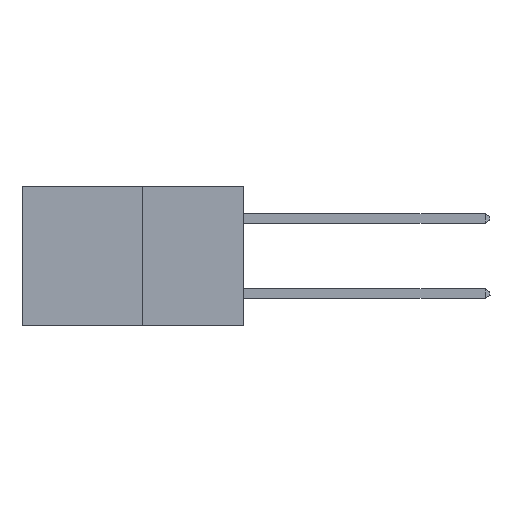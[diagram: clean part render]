
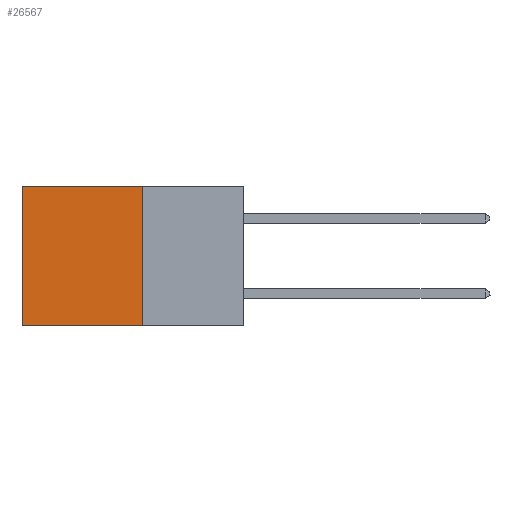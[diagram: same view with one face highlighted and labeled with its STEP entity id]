
A CAD part, left-side view. The second image highlights one B-rep face of the part: STEP entity #26567.
In plain terms, the highlighted planar face has unit normal (-1, 0, 0).
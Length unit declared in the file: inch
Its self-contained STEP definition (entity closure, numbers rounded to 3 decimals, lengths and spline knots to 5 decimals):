
#114 = FACE_OUTER_BOUND ( 'NONE', #4023, .T. ) ;
#554 = EDGE_CURVE ( 'NONE', #22912, #1850, #18819, .T. ) ;
#1509 = CARTESIAN_POINT ( 'NONE',  ( 0.277, 0.59, -0.37 ) ) ;
#1777 = CARTESIAN_POINT ( 'NONE',  ( 0.277, 0.27, -0.37 ) ) ;
#1818 = VERTEX_POINT ( 'NONE', #24391 ) ;
#1850 = VERTEX_POINT ( 'NONE', #26605 ) ;
#2581 = ORIENTED_EDGE ( 'NONE', *, *, #26388, .T. ) ;
#4023 = EDGE_LOOP ( 'NONE', ( #2581, #30947, #9763, #32124 ) ) ;
#4091 = VERTEX_POINT ( 'NONE', #1777 ) ;
#4722 = DIRECTION ( 'NONE',  ( 1., 0., 0. ) ) ;
#4910 = VECTOR ( 'NONE', #6625, 39.37008 ) ;
#5679 = CARTESIAN_POINT ( 'NONE',  ( 0.277, 0.27, 0. ) ) ;
#6625 = DIRECTION ( 'NONE',  ( 0., 0., -1. ) ) ;
#9743 = CARTESIAN_POINT ( 'NONE',  ( 0.277, 0.27, -0.37 ) ) ;
#9763 = ORIENTED_EDGE ( 'NONE', *, *, #24203, .F. ) ;
#10411 = VECTOR ( 'NONE', #16043, 39.37008 ) ;
#11686 = LINE ( 'NONE', #1509, #4910 ) ;
#16043 = DIRECTION ( 'NONE',  ( 0., 0., -1. ) ) ;
#17228 = AXIS2_PLACEMENT_3D ( 'NONE', #9743, #4722, #22443 ) ;
#18179 = DIRECTION ( 'NONE',  ( 0., 1., 0. ) ) ;
#18819 = LINE ( 'NONE', #5679, #31328 ) ;
#18998 = VECTOR ( 'NONE', #21458, 39.37008 ) ;
#21458 = DIRECTION ( 'NONE',  ( 0., 1., 0. ) ) ;
#22443 = DIRECTION ( 'NONE',  ( 0., 0., -1. ) ) ;
#22912 = VERTEX_POINT ( 'NONE', #24049 ) ;
#23049 = LINE ( 'NONE', #26058, #10411 ) ;
#24049 = CARTESIAN_POINT ( 'NONE',  ( 0.277, 0.27, 0. ) ) ;
#24203 = EDGE_CURVE ( 'NONE', #22912, #4091, #23049, .T. ) ;
#24391 = CARTESIAN_POINT ( 'NONE',  ( 0.277, 0.59, -0.37 ) ) ;
#25690 = LINE ( 'NONE', #31341, #18998 ) ;
#26058 = CARTESIAN_POINT ( 'NONE',  ( 0.277, 0.27, -0.37 ) ) ;
#26388 = EDGE_CURVE ( 'NONE', #1850, #1818, #11686, .T. ) ;
#26567 = ADVANCED_FACE ( 'NONE', ( #114 ), #27343, .F. ) ;
#26605 = CARTESIAN_POINT ( 'NONE',  ( 0.277, 0.59, 0. ) ) ;
#27343 = PLANE ( 'NONE',  #17228 ) ;
#29272 = EDGE_CURVE ( 'NONE', #4091, #1818, #25690, .T. ) ;
#30947 = ORIENTED_EDGE ( 'NONE', *, *, #29272, .F. ) ;
#31328 = VECTOR ( 'NONE', #18179, 39.37008 ) ;
#31341 = CARTESIAN_POINT ( 'NONE',  ( 0.277, 0.27, -0.37 ) ) ;
#32124 = ORIENTED_EDGE ( 'NONE', *, *, #554, .T. ) ;
